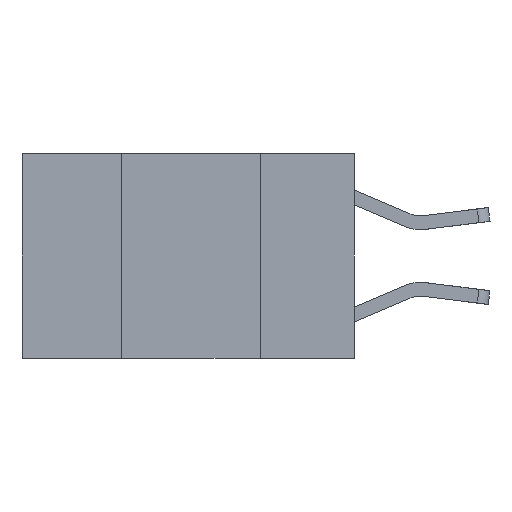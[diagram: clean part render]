
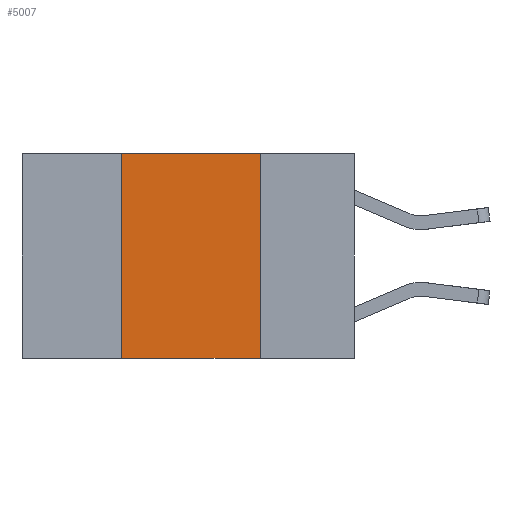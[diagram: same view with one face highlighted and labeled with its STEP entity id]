
A CAD part, left-side view. The second image highlights one B-rep face of the part: STEP entity #5007.
In plain terms, the highlighted planar face has unit normal (-1, 0, 0).
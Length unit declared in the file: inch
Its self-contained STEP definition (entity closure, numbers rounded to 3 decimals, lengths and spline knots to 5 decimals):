
#458 = VERTEX_POINT ( 'NONE', #7496 ) ;
#601 = DIRECTION ( 'NONE',  ( 0., 0., -1. ) ) ;
#712 = LINE ( 'NONE', #5810, #9211 ) ;
#821 = DIRECTION ( 'NONE',  ( 1., 0., 0. ) ) ;
#823 = ORIENTED_EDGE ( 'NONE', *, *, #2087, .F. ) ;
#1729 = EDGE_CURVE ( 'NONE', #458, #6259, #712, .T. ) ;
#2001 = EDGE_CURVE ( 'NONE', #6259, #7733, #6861, .T. ) ;
#2087 = EDGE_CURVE ( 'NONE', #7733, #8434, #3712, .T. ) ;
#2454 = CARTESIAN_POINT ( 'NONE',  ( 0., 0.17, 0. ) ) ;
#2918 = VECTOR ( 'NONE', #8278, 39.37008 ) ;
#3175 = LINE ( 'NONE', #7450, #2918 ) ;
#3712 = LINE ( 'NONE', #6192, #7737 ) ;
#3793 = AXIS2_PLACEMENT_3D ( 'NONE', #10740, #821, #6547 ) ;
#4441 = FACE_OUTER_BOUND ( 'NONE', #10550, .T. ) ;
#4948 = PLANE ( 'NONE',  #3793 ) ;
#4994 = DIRECTION ( 'NONE',  ( 0., 0., 1. ) ) ;
#5007 = ADVANCED_FACE ( 'NONE', ( #4441 ), #4948, .F. ) ;
#5507 = CARTESIAN_POINT ( 'NONE',  ( 0., 0.6, 0. ) ) ;
#5752 = CARTESIAN_POINT ( 'NONE',  ( 0., 0.17, -0.37 ) ) ;
#5810 = CARTESIAN_POINT ( 'NONE',  ( 0., 0.42, 0. ) ) ;
#6192 = CARTESIAN_POINT ( 'NONE',  ( 0., 0.17, 0. ) ) ;
#6259 = VERTEX_POINT ( 'NONE', #10676 ) ;
#6547 = DIRECTION ( 'NONE',  ( 0., 0., -1. ) ) ;
#6861 = LINE ( 'NONE', #5507, #8814 ) ;
#7450 = CARTESIAN_POINT ( 'NONE',  ( 0., 0.6, -0.37 ) ) ;
#7496 = CARTESIAN_POINT ( 'NONE',  ( 0., 0.42, -0.37 ) ) ;
#7733 = VERTEX_POINT ( 'NONE', #2454 ) ;
#7737 = VECTOR ( 'NONE', #601, 39.37008 ) ;
#8278 = DIRECTION ( 'NONE',  ( 0., -1., 0. ) ) ;
#8434 = VERTEX_POINT ( 'NONE', #5752 ) ;
#8814 = VECTOR ( 'NONE', #9489, 39.37008 ) ;
#9211 = VECTOR ( 'NONE', #4994, 39.37008 ) ;
#9489 = DIRECTION ( 'NONE',  ( 0., -1., 0. ) ) ;
#9761 = ORIENTED_EDGE ( 'NONE', *, *, #10075, .T. ) ;
#10075 = EDGE_CURVE ( 'NONE', #458, #8434, #3175, .T. ) ;
#10273 = ORIENTED_EDGE ( 'NONE', *, *, #1729, .F. ) ;
#10550 = EDGE_LOOP ( 'NONE', ( #823, #10688, #10273, #9761 ) ) ;
#10676 = CARTESIAN_POINT ( 'NONE',  ( 0., 0.42, 0. ) ) ;
#10688 = ORIENTED_EDGE ( 'NONE', *, *, #2001, .F. ) ;
#10740 = CARTESIAN_POINT ( 'NONE',  ( 0., 0.6, 0. ) ) ;
